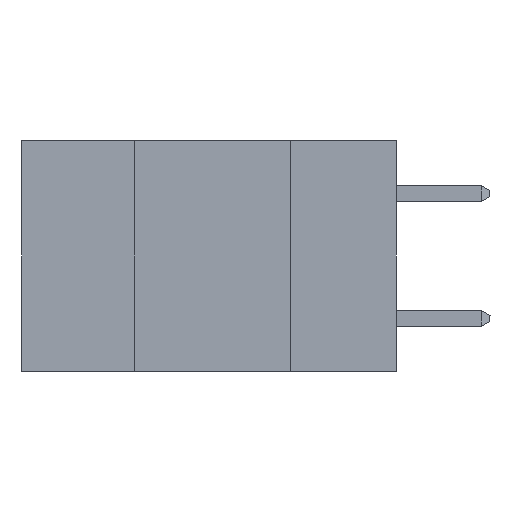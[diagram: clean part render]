
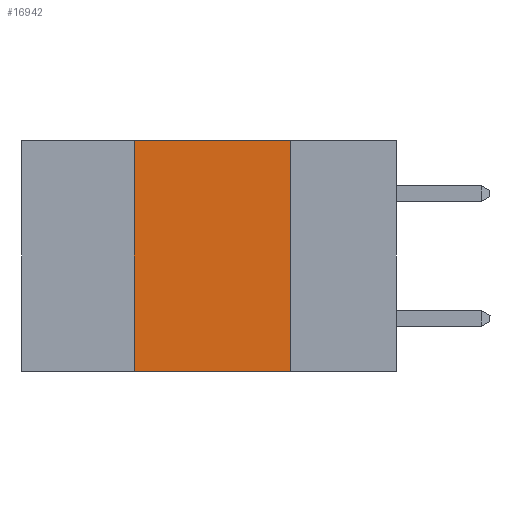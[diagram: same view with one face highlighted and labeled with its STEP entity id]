
A CAD part, left-side view. The second image highlights one B-rep face of the part: STEP entity #16942.
In plain terms, the highlighted planar face has unit normal (-1, 0, 0).
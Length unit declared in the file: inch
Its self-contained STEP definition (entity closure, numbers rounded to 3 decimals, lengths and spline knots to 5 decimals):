
#1026 = DIRECTION ( 'NONE',  ( 0., 0., -1. ) ) ;
#3002 = VECTOR ( 'NONE', #10352, 39.37008 ) ;
#3818 = CARTESIAN_POINT ( 'NONE',  ( 0., 0.42, -0.37 ) ) ;
#4484 = EDGE_CURVE ( 'NONE', #7594, #11049, #21213, .T. ) ;
#4528 = DIRECTION ( 'NONE',  ( 0., -1., 0. ) ) ;
#5114 = CARTESIAN_POINT ( 'NONE',  ( 0., 0.6, -0.37 ) ) ;
#5679 = EDGE_CURVE ( 'NONE', #7594, #21899, #8361, .T. ) ;
#6307 = CARTESIAN_POINT ( 'NONE',  ( 0., 0.6, 0. ) ) ;
#7071 = EDGE_LOOP ( 'NONE', ( #18273, #7725, #20567, #11442 ) ) ;
#7340 = VECTOR ( 'NONE', #4528, 39.37008 ) ;
#7594 = VERTEX_POINT ( 'NONE', #3818 ) ;
#7725 = ORIENTED_EDGE ( 'NONE', *, *, #8023, .F. ) ;
#8023 = EDGE_CURVE ( 'NONE', #21899, #15966, #8033, .T. ) ;
#8033 = LINE ( 'NONE', #8802, #20827 ) ;
#8196 = FACE_OUTER_BOUND ( 'NONE', #7071, .T. ) ;
#8361 = LINE ( 'NONE', #17847, #12297 ) ;
#8647 = CARTESIAN_POINT ( 'NONE',  ( 0., 0.17, -0.37 ) ) ;
#8802 = CARTESIAN_POINT ( 'NONE',  ( 0., 0.6, 0. ) ) ;
#9165 = EDGE_CURVE ( 'NONE', #15966, #11049, #12176, .T. ) ;
#9477 = DIRECTION ( 'NONE',  ( 0., 0., 1. ) ) ;
#10352 = DIRECTION ( 'NONE',  ( 0., 0., -1. ) ) ;
#10488 = DIRECTION ( 'NONE',  ( 0., -1., 0. ) ) ;
#11049 = VERTEX_POINT ( 'NONE', #20198 ) ;
#11433 = DIRECTION ( 'NONE',  ( 1., 0., 0. ) ) ;
#11442 = ORIENTED_EDGE ( 'NONE', *, *, #4484, .T. ) ;
#12176 = LINE ( 'NONE', #8647, #3002 ) ;
#12297 = VECTOR ( 'NONE', #9477, 39.37008 ) ;
#13822 = CARTESIAN_POINT ( 'NONE',  ( 0., 0.17, 0. ) ) ;
#14353 = AXIS2_PLACEMENT_3D ( 'NONE', #6307, #11433, #1026 ) ;
#14720 = CARTESIAN_POINT ( 'NONE',  ( 0., 0.42, 0. ) ) ;
#15966 = VERTEX_POINT ( 'NONE', #13822 ) ;
#16942 = ADVANCED_FACE ( 'NONE', ( #8196 ), #19761, .F. ) ;
#17847 = CARTESIAN_POINT ( 'NONE',  ( 0., 0.42, -0.37 ) ) ;
#18273 = ORIENTED_EDGE ( 'NONE', *, *, #9165, .F. ) ;
#19761 = PLANE ( 'NONE',  #14353 ) ;
#20198 = CARTESIAN_POINT ( 'NONE',  ( 0., 0.17, -0.37 ) ) ;
#20567 = ORIENTED_EDGE ( 'NONE', *, *, #5679, .F. ) ;
#20827 = VECTOR ( 'NONE', #10488, 39.37008 ) ;
#21213 = LINE ( 'NONE', #5114, #7340 ) ;
#21899 = VERTEX_POINT ( 'NONE', #14720 ) ;
